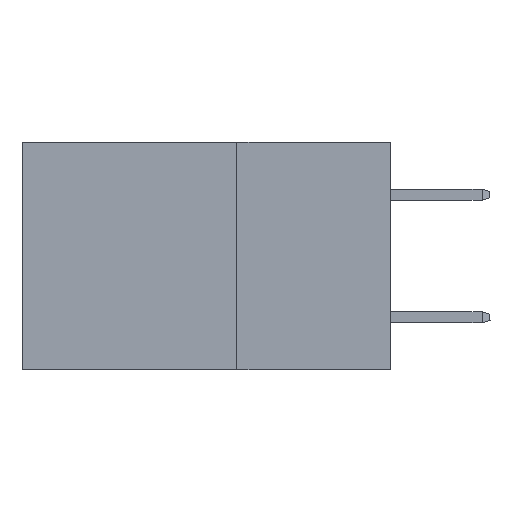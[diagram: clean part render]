
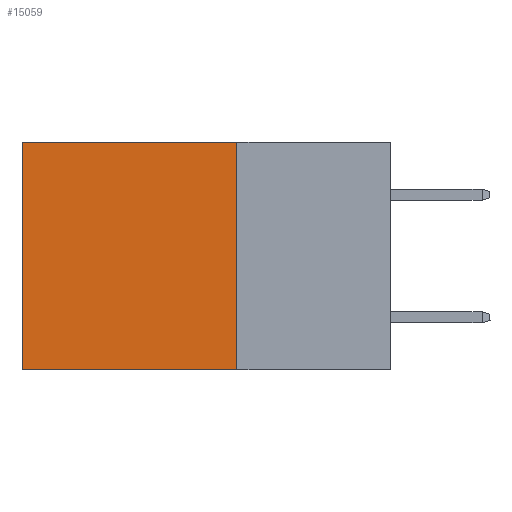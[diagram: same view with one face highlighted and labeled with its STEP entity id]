
A CAD part, left-side view. The second image highlights one B-rep face of the part: STEP entity #15059.
In plain terms, the highlighted planar face has unit normal (-1, 0, 0).
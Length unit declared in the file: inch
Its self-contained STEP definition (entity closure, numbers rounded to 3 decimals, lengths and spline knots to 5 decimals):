
#2112 = VERTEX_POINT ( 'NONE', #19562 ) ;
#3087 = FACE_OUTER_BOUND ( 'NONE', #23837, .T. ) ;
#3135 = ORIENTED_EDGE ( 'NONE', *, *, #3958, .F. ) ;
#3958 = EDGE_CURVE ( 'NONE', #8918, #19553, #37795, .T. ) ;
#8918 = VERTEX_POINT ( 'NONE', #21645 ) ;
#10570 = ORIENTED_EDGE ( 'NONE', *, *, #25150, .T. ) ;
#12076 = CARTESIAN_POINT ( 'NONE',  ( 0.2875, 0.25, 0. ) ) ;
#13815 = EDGE_CURVE ( 'NONE', #42879, #8918, #31171, .T. ) ;
#13977 = VECTOR ( 'NONE', #25851, 39.37008 ) ;
#15059 = ADVANCED_FACE ( 'NONE', ( #3087 ), #21532, .F. ) ;
#15675 = CARTESIAN_POINT ( 'NONE',  ( 0.2875, 0.25, 0. ) ) ;
#18052 = DIRECTION ( 'NONE',  ( 1., 0., 0. ) ) ;
#19553 = VERTEX_POINT ( 'NONE', #23533 ) ;
#19562 = CARTESIAN_POINT ( 'NONE',  ( 0.2875, 0.6, 0. ) ) ;
#20245 = VECTOR ( 'NONE', #27459, 39.37008 ) ;
#20418 = ORIENTED_EDGE ( 'NONE', *, *, #24760, .T. ) ;
#21532 = PLANE ( 'NONE',  #43998 ) ;
#21645 = CARTESIAN_POINT ( 'NONE',  ( 0.2875, 0.25, -0.37 ) ) ;
#23533 = CARTESIAN_POINT ( 'NONE',  ( 0.2875, 0.6, -0.37 ) ) ;
#23837 = EDGE_LOOP ( 'NONE', ( #20418, #3135, #23960, #10570 ) ) ;
#23960 = ORIENTED_EDGE ( 'NONE', *, *, #13815, .F. ) ;
#24760 = EDGE_CURVE ( 'NONE', #2112, #19553, #29878, .T. ) ;
#25150 = EDGE_CURVE ( 'NONE', #42879, #2112, #34345, .T. ) ;
#25851 = DIRECTION ( 'NONE',  ( 0., 1., 0. ) ) ;
#26387 = CARTESIAN_POINT ( 'NONE',  ( 0.2875, 0.25, -0.37 ) ) ;
#27459 = DIRECTION ( 'NONE',  ( 0., 0., -1. ) ) ;
#29878 = LINE ( 'NONE', #30937, #20245 ) ;
#30937 = CARTESIAN_POINT ( 'NONE',  ( 0.2875, 0.6, 0. ) ) ;
#31171 = LINE ( 'NONE', #12076, #44395 ) ;
#33081 = CARTESIAN_POINT ( 'NONE',  ( 0.2875, 0.25, 0. ) ) ;
#33632 = DIRECTION ( 'NONE',  ( 0., 1., 0. ) ) ;
#34345 = LINE ( 'NONE', #33081, #13977 ) ;
#36677 = VECTOR ( 'NONE', #33632, 39.37008 ) ;
#37795 = LINE ( 'NONE', #26387, #36677 ) ;
#39570 = CARTESIAN_POINT ( 'NONE',  ( 0.2875, 0.25, 0. ) ) ;
#40854 = DIRECTION ( 'NONE',  ( 0., 0., -1. ) ) ;
#42879 = VERTEX_POINT ( 'NONE', #15675 ) ;
#43073 = DIRECTION ( 'NONE',  ( 0., 0., -1. ) ) ;
#43998 = AXIS2_PLACEMENT_3D ( 'NONE', #39570, #18052, #43073 ) ;
#44395 = VECTOR ( 'NONE', #40854, 39.37008 ) ;
